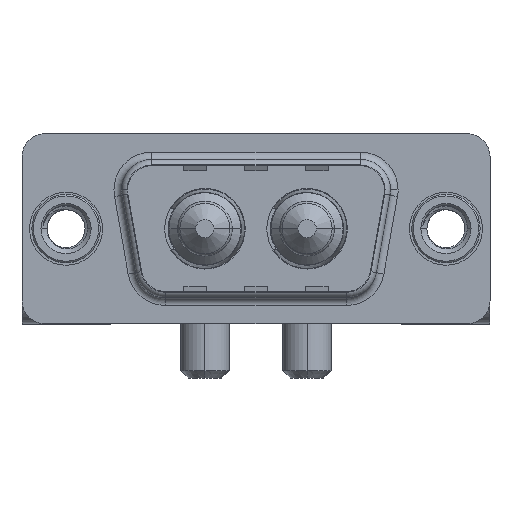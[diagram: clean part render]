
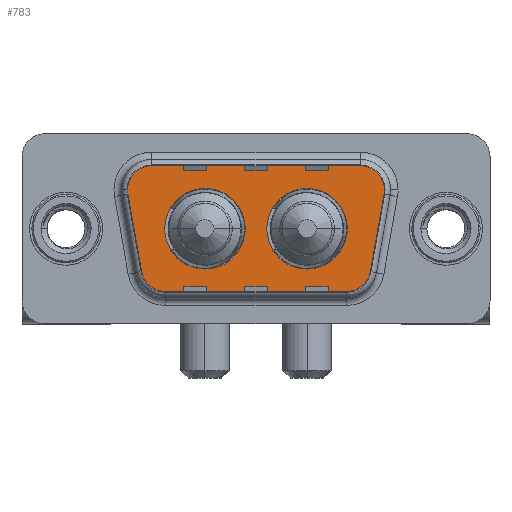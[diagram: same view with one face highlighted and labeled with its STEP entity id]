
A CAD part, top view. The second image highlights one B-rep face of the part: STEP entity #783.
In plain terms, the highlighted planar face has unit normal (0, 0, 1).
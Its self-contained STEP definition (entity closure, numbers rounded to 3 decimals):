
#54 = DIRECTION ( 'NONE',  ( 0., 0., 1. ) ) ;
#125 = CARTESIAN_POINT ( 'NONE',  ( 15.86, 0., 0. ) ) ;
#139 = DIRECTION ( 'NONE',  ( 0., 0., 1. ) ) ;
#330 = VERTEX_POINT ( 'NONE', #3914 ) ;
#405 = DIRECTION ( 'NONE',  ( 0., 0., 1. ) ) ;
#483 = EDGE_CURVE ( 'NONE', #12334, #3514, #10673, .T. ) ;
#490 = CARTESIAN_POINT ( 'NONE',  ( 21.534, 2.553, 0. ) ) ;
#509 = ORIENTED_EDGE ( 'NONE', *, *, #7553, .T. ) ;
#551 = VERTEX_POINT ( 'NONE', #4244 ) ;
#661 = VECTOR ( 'NONE', #5770, 1000. ) ;
#671 = LINE ( 'NONE', #2935, #13494 ) ;
#677 = AXIS2_PLACEMENT_3D ( 'NONE', #3669, #405, #6928 ) ;
#783 = ADVANCED_FACE ( 'NONE', ( #3462, #11155, #10868 ), #7719, .T. ) ;
#787 = DIRECTION ( 'NONE',  ( 1., 0., 0. ) ) ;
#790 = CARTESIAN_POINT ( 'NONE',  ( 6.459, -4.9, 0. ) ) ;
#922 = DIRECTION ( 'NONE',  ( 1., 0., 0. ) ) ;
#1073 = DIRECTION ( 'NONE',  ( 0.174, 0.985, 0. ) ) ;
#1434 = DIRECTION ( 'NONE',  ( -1., 0., 0. ) ) ;
#1581 = CIRCLE ( 'NONE', #13634, 2.65 ) ;
#1751 = EDGE_CURVE ( 'NONE', #9506, #4679, #11252, .T. ) ;
#1834 = EDGE_LOOP ( 'NONE', ( #11282, #7281 ) ) ;
#2203 = DIRECTION ( 'NONE',  ( 0., 0., 1. ) ) ;
#2381 = DIRECTION ( 'NONE',  ( -1., 0., 0. ) ) ;
#2525 = EDGE_LOOP ( 'NONE', ( #8506, #9519 ) ) ;
#2827 = DIRECTION ( 'NONE',  ( 0., 0., 1. ) ) ;
#2935 = CARTESIAN_POINT ( 'NONE',  ( 3.466, 2.553, 0. ) ) ;
#2945 = AXIS2_PLACEMENT_3D ( 'NONE', #12725, #2827, #2966 ) ;
#2966 = DIRECTION ( 'NONE',  ( 1., 0., 0. ) ) ;
#2978 = DIRECTION ( 'NONE',  ( 0., 0., 1. ) ) ;
#3151 = CIRCLE ( 'NONE', #11105, 2.65 ) ;
#3462 = FACE_BOUND ( 'NONE', #1834, .T. ) ;
#3514 = VERTEX_POINT ( 'NONE', #11672 ) ;
#3669 = CARTESIAN_POINT ( 'NONE',  ( 5.436, 2.9, 0. ) ) ;
#3681 = AXIS2_PLACEMENT_3D ( 'NONE', #5561, #7776, #2381 ) ;
#3737 = ORIENTED_EDGE ( 'NONE', *, *, #8870, .T. ) ;
#3860 = DIRECTION ( 'NONE',  ( 0.174, -0.985, 0. ) ) ;
#3914 = CARTESIAN_POINT ( 'NONE',  ( 6.49, 0., 0. ) ) ;
#3980 = DIRECTION ( 'NONE',  ( 0., 0., 1. ) ) ;
#4022 = AXIS2_PLACEMENT_3D ( 'NONE', #13597, #2978, #12802 ) ;
#4046 = CARTESIAN_POINT ( 'NONE',  ( 19.564, 4.9, 0. ) ) ;
#4064 = DIRECTION ( 'NONE',  ( 1., 0., 0. ) ) ;
#4195 = AXIS2_PLACEMENT_3D ( 'NONE', #9957, #8883, #1434 ) ;
#4244 = CARTESIAN_POINT ( 'NONE',  ( 3.466, 2.553, 0. ) ) ;
#4386 = DIRECTION ( 'NONE',  ( 1., 0., 0. ) ) ;
#4447 = DIRECTION ( 'NONE',  ( 1., 0., 0. ) ) ;
#4678 = CARTESIAN_POINT ( 'NONE',  ( 20.511, -3.247, 0. ) ) ;
#4679 = VERTEX_POINT ( 'NONE', #4046 ) ;
#4692 = EDGE_CURVE ( 'NONE', #13639, #9562, #3151, .T. ) ;
#4784 = LINE ( 'NONE', #9977, #661 ) ;
#5072 = VECTOR ( 'NONE', #922, 1000. ) ;
#5179 = ORIENTED_EDGE ( 'NONE', *, *, #9533, .T. ) ;
#5183 = AXIS2_PLACEMENT_3D ( 'NONE', #9322, #8330, #12634 ) ;
#5220 = EDGE_CURVE ( 'NONE', #330, #6015, #6550, .T. ) ;
#5561 = CARTESIAN_POINT ( 'NONE',  ( 19.564, 2.9, 0. ) ) ;
#5770 = DIRECTION ( 'NONE',  ( -1., 0., 0. ) ) ;
#5972 = ORIENTED_EDGE ( 'NONE', *, *, #1751, .T. ) ;
#6015 = VERTEX_POINT ( 'NONE', #6956 ) ;
#6375 = AXIS2_PLACEMENT_3D ( 'NONE', #10821, #2203, #4064 ) ;
#6404 = VERTEX_POINT ( 'NONE', #490 ) ;
#6550 = CIRCLE ( 'NONE', #2945, 2.65 ) ;
#6801 = CARTESIAN_POINT ( 'NONE',  ( 18.541, -2.9, 0. ) ) ;
#6928 = DIRECTION ( 'NONE',  ( 1., 0., 0. ) ) ;
#6956 = CARTESIAN_POINT ( 'NONE',  ( 11.79, 0., 0. ) ) ;
#7095 = CARTESIAN_POINT ( 'NONE',  ( 21.564, 2.9, 0. ) ) ;
#7281 = ORIENTED_EDGE ( 'NONE', *, *, #12988, .F. ) ;
#7426 = ORIENTED_EDGE ( 'NONE', *, *, #13139, .T. ) ;
#7553 = EDGE_CURVE ( 'NONE', #12870, #6404, #13767, .T. ) ;
#7719 = PLANE ( 'NONE',  #13046 ) ;
#7776 = DIRECTION ( 'NONE',  ( 0., 0., 1. ) ) ;
#7905 = CARTESIAN_POINT ( 'NONE',  ( 18.51, 0., 0. ) ) ;
#8257 = EDGE_CURVE ( 'NONE', #6404, #9506, #10942, .T. ) ;
#8330 = DIRECTION ( 'NONE',  ( 0., 0., 1. ) ) ;
#8377 = CIRCLE ( 'NONE', #677, 2. ) ;
#8418 = CIRCLE ( 'NONE', #6375, 2.65 ) ;
#8461 = CARTESIAN_POINT ( 'NONE',  ( 5.436, 4.9, 0. ) ) ;
#8506 = ORIENTED_EDGE ( 'NONE', *, *, #9113, .F. ) ;
#8870 = EDGE_CURVE ( 'NONE', #551, #13582, #671, .T. ) ;
#8883 = DIRECTION ( 'NONE',  ( 0., 0., 1. ) ) ;
#9113 = EDGE_CURVE ( 'NONE', #6015, #330, #8418, .T. ) ;
#9322 = CARTESIAN_POINT ( 'NONE',  ( 6.459, -2.9, 0. ) ) ;
#9506 = VERTEX_POINT ( 'NONE', #7095 ) ;
#9519 = ORIENTED_EDGE ( 'NONE', *, *, #5220, .F. ) ;
#9533 = EDGE_CURVE ( 'NONE', #3514, #12870, #10150, .T. ) ;
#9562 = VERTEX_POINT ( 'NONE', #13739 ) ;
#9646 = ORIENTED_EDGE ( 'NONE', *, *, #8257, .T. ) ;
#9748 = CARTESIAN_POINT ( 'NONE',  ( 6.459, -4.9, 0. ) ) ;
#9957 = CARTESIAN_POINT ( 'NONE',  ( 19.564, 2.9, 0. ) ) ;
#9977 = CARTESIAN_POINT ( 'NONE',  ( 5.436, 4.9, 0. ) ) ;
#10054 = VERTEX_POINT ( 'NONE', #8461 ) ;
#10150 = CIRCLE ( 'NONE', #4022, 2. ) ;
#10195 = CARTESIAN_POINT ( 'NONE',  ( 4.489, -3.247, 0. ) ) ;
#10673 = LINE ( 'NONE', #790, #5072 ) ;
#10721 = ORIENTED_EDGE ( 'NONE', *, *, #11997, .T. ) ;
#10821 = CARTESIAN_POINT ( 'NONE',  ( 9.14, 0., 0. ) ) ;
#10868 = FACE_OUTER_BOUND ( 'NONE', #11560, .T. ) ;
#10942 = CIRCLE ( 'NONE', #3681, 2. ) ;
#11105 = AXIS2_PLACEMENT_3D ( 'NONE', #13538, #3980, #787 ) ;
#11155 = FACE_BOUND ( 'NONE', #2525, .T. ) ;
#11219 = ORIENTED_EDGE ( 'NONE', *, *, #12262, .T. ) ;
#11252 = CIRCLE ( 'NONE', #4195, 2. ) ;
#11282 = ORIENTED_EDGE ( 'NONE', *, *, #4692, .F. ) ;
#11334 = CIRCLE ( 'NONE', #5183, 2. ) ;
#11560 = EDGE_LOOP ( 'NONE', ( #5179, #509, #9646, #5972, #10721, #7426, #3737, #11219, #13762 ) ) ;
#11672 = CARTESIAN_POINT ( 'NONE',  ( 18.541, -4.9, 0. ) ) ;
#11686 = CARTESIAN_POINT ( 'NONE',  ( 21.534, 2.553, 0. ) ) ;
#11885 = VECTOR ( 'NONE', #1073, 1000. ) ;
#11997 = EDGE_CURVE ( 'NONE', #4679, #10054, #4784, .T. ) ;
#12262 = EDGE_CURVE ( 'NONE', #13582, #12334, #11334, .T. ) ;
#12334 = VERTEX_POINT ( 'NONE', #9748 ) ;
#12634 = DIRECTION ( 'NONE',  ( -1., 0., 0. ) ) ;
#12725 = CARTESIAN_POINT ( 'NONE',  ( 9.14, 0., 0. ) ) ;
#12802 = DIRECTION ( 'NONE',  ( 1., 0., 0. ) ) ;
#12870 = VERTEX_POINT ( 'NONE', #4678 ) ;
#12988 = EDGE_CURVE ( 'NONE', #9562, #13639, #1581, .T. ) ;
#13046 = AXIS2_PLACEMENT_3D ( 'NONE', #6801, #139, #4386 ) ;
#13139 = EDGE_CURVE ( 'NONE', #10054, #551, #8377, .T. ) ;
#13494 = VECTOR ( 'NONE', #3860, 1000. ) ;
#13538 = CARTESIAN_POINT ( 'NONE',  ( 15.86, 0., 0. ) ) ;
#13582 = VERTEX_POINT ( 'NONE', #10195 ) ;
#13597 = CARTESIAN_POINT ( 'NONE',  ( 18.541, -2.9, 0. ) ) ;
#13634 = AXIS2_PLACEMENT_3D ( 'NONE', #125, #54, #4447 ) ;
#13639 = VERTEX_POINT ( 'NONE', #7905 ) ;
#13739 = CARTESIAN_POINT ( 'NONE',  ( 13.21, 0., 0. ) ) ;
#13762 = ORIENTED_EDGE ( 'NONE', *, *, #483, .T. ) ;
#13767 = LINE ( 'NONE', #11686, #11885 ) ;
